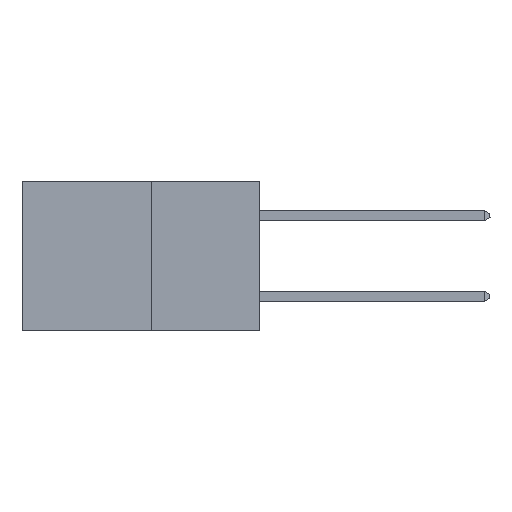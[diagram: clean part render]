
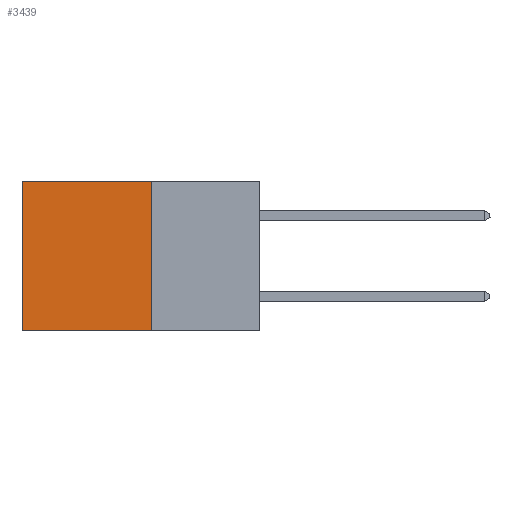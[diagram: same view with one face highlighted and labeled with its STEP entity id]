
A CAD part, left-side view. The second image highlights one B-rep face of the part: STEP entity #3439.
In plain terms, the highlighted planar face has unit normal (-1, 0, 0).
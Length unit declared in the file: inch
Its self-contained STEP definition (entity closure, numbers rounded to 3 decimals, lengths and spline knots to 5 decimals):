
#804 = CARTESIAN_POINT ( 'NONE',  ( 0.277, 0.27, 0. ) ) ;
#829 = DIRECTION ( 'NONE',  ( 0., 1., 0. ) ) ;
#832 = CARTESIAN_POINT ( 'NONE',  ( 0.277, 0.27, -0.37 ) ) ;
#1387 = CARTESIAN_POINT ( 'NONE',  ( 0.277, 0.59, 0. ) ) ;
#1839 = PLANE ( 'NONE',  #4863 ) ;
#2301 = EDGE_CURVE ( 'NONE', #13060, #3120, #15419, .T. ) ;
#2377 = ORIENTED_EDGE ( 'NONE', *, *, #2301, .T. ) ;
#2727 = ORIENTED_EDGE ( 'NONE', *, *, #6023, .T. ) ;
#3120 = VERTEX_POINT ( 'NONE', #10954 ) ;
#3439 = ADVANCED_FACE ( 'NONE', ( #15408 ), #1839, .F. ) ;
#3555 = VECTOR ( 'NONE', #14463, 39.37008 ) ;
#3659 = CARTESIAN_POINT ( 'NONE',  ( 0.277, 0.59, -0.37 ) ) ;
#3899 = ORIENTED_EDGE ( 'NONE', *, *, #9065, .F. ) ;
#4863 = AXIS2_PLACEMENT_3D ( 'NONE', #13794, #6702, #11493 ) ;
#5125 = EDGE_CURVE ( 'NONE', #7391, #12723, #10435, .T. ) ;
#5302 = DIRECTION ( 'NONE',  ( 0., 0., -1. ) ) ;
#5373 = ORIENTED_EDGE ( 'NONE', *, *, #5125, .F. ) ;
#5690 = CARTESIAN_POINT ( 'NONE',  ( 0.277, 0.27, -0.37 ) ) ;
#6023 = EDGE_CURVE ( 'NONE', #7391, #13060, #12248, .T. ) ;
#6600 = EDGE_LOOP ( 'NONE', ( #2377, #3899, #5373, #2727 ) ) ;
#6702 = DIRECTION ( 'NONE',  ( 1., 0., 0. ) ) ;
#7391 = VERTEX_POINT ( 'NONE', #804 ) ;
#9065 = EDGE_CURVE ( 'NONE', #12723, #3120, #11224, .T. ) ;
#10435 = LINE ( 'NONE', #14592, #3555 ) ;
#10954 = CARTESIAN_POINT ( 'NONE',  ( 0.277, 0.59, -0.37 ) ) ;
#11224 = LINE ( 'NONE', #5690, #11608 ) ;
#11493 = DIRECTION ( 'NONE',  ( 0., 0., -1. ) ) ;
#11608 = VECTOR ( 'NONE', #829, 39.37008 ) ;
#12248 = LINE ( 'NONE', #12353, #15105 ) ;
#12353 = CARTESIAN_POINT ( 'NONE',  ( 0.277, 0.27, 0. ) ) ;
#12568 = VECTOR ( 'NONE', #5302, 39.37008 ) ;
#12723 = VERTEX_POINT ( 'NONE', #832 ) ;
#12971 = DIRECTION ( 'NONE',  ( 0., 1., 0. ) ) ;
#13060 = VERTEX_POINT ( 'NONE', #1387 ) ;
#13794 = CARTESIAN_POINT ( 'NONE',  ( 0.277, 0.27, -0.37 ) ) ;
#14463 = DIRECTION ( 'NONE',  ( 0., 0., -1. ) ) ;
#14592 = CARTESIAN_POINT ( 'NONE',  ( 0.277, 0.27, -0.37 ) ) ;
#15105 = VECTOR ( 'NONE', #12971, 39.37008 ) ;
#15408 = FACE_OUTER_BOUND ( 'NONE', #6600, .T. ) ;
#15419 = LINE ( 'NONE', #3659, #12568 ) ;
